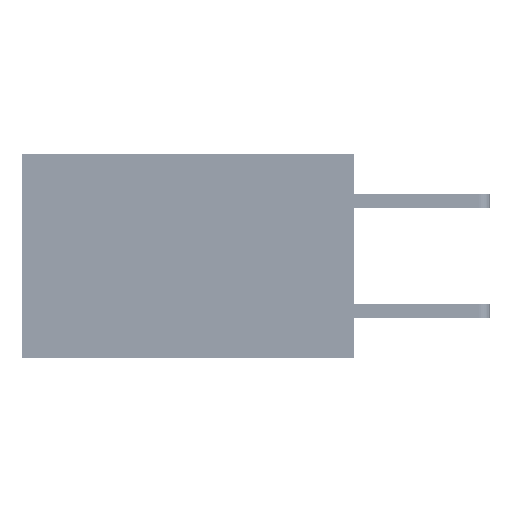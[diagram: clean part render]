
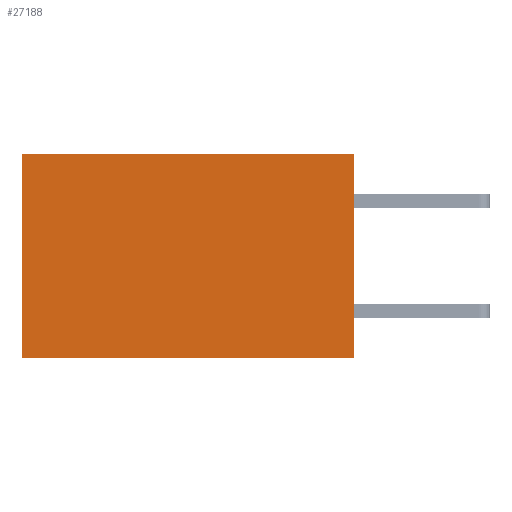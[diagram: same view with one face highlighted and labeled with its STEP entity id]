
A CAD part, left-side view. The second image highlights one B-rep face of the part: STEP entity #27188.
In plain terms, the highlighted planar face has unit normal (-1, 0, 0).
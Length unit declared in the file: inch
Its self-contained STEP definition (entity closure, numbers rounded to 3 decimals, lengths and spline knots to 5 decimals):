
#1308 = VERTEX_POINT ( 'NONE', #6621 ) ;
#3242 = DIRECTION ( 'NONE',  ( 0., 1., 0. ) ) ;
#3298 = VECTOR ( 'NONE', #3719, 39.37008 ) ;
#3719 = DIRECTION ( 'NONE',  ( 0., 1., 0. ) ) ;
#4143 = LINE ( 'NONE', #37745, #36942 ) ;
#4785 = VECTOR ( 'NONE', #3242, 39.37008 ) ;
#5758 = PLANE ( 'NONE',  #33249 ) ;
#6358 = LINE ( 'NONE', #19560, #4785 ) ;
#6621 = CARTESIAN_POINT ( 'NONE',  ( 0.2875, 0., 0. ) ) ;
#7656 = ORIENTED_EDGE ( 'NONE', *, *, #20569, .F. ) ;
#8825 = ORIENTED_EDGE ( 'NONE', *, *, #31269, .F. ) ;
#9727 = CARTESIAN_POINT ( 'NONE',  ( 0.2875, 0.6, -0.37 ) ) ;
#12631 = CARTESIAN_POINT ( 'NONE',  ( 0.2875, 0., 0. ) ) ;
#16343 = FACE_OUTER_BOUND ( 'NONE', #20433, .T. ) ;
#17646 = LINE ( 'NONE', #33254, #3298 ) ;
#17921 = EDGE_CURVE ( 'NONE', #32695, #18899, #24446, .T. ) ;
#18115 = DIRECTION ( 'NONE',  ( 0., 0., -1. ) ) ;
#18247 = VECTOR ( 'NONE', #21231, 39.37008 ) ;
#18899 = VERTEX_POINT ( 'NONE', #9727 ) ;
#19560 = CARTESIAN_POINT ( 'NONE',  ( 0.2875, 0., 0. ) ) ;
#20433 = EDGE_LOOP ( 'NONE', ( #25831, #8825, #7656, #35516 ) ) ;
#20569 = EDGE_CURVE ( 'NONE', #1308, #21246, #4143, .T. ) ;
#21231 = DIRECTION ( 'NONE',  ( 0., 0., -1. ) ) ;
#21246 = VERTEX_POINT ( 'NONE', #38425 ) ;
#22358 = DIRECTION ( 'NONE',  ( 1., 0., 0. ) ) ;
#24446 = LINE ( 'NONE', #40715, #18247 ) ;
#25831 = ORIENTED_EDGE ( 'NONE', *, *, #17921, .T. ) ;
#27188 = ADVANCED_FACE ( 'NONE', ( #16343 ), #5758, .F. ) ;
#31269 = EDGE_CURVE ( 'NONE', #21246, #18899, #17646, .T. ) ;
#31753 = EDGE_CURVE ( 'NONE', #1308, #32695, #6358, .T. ) ;
#32695 = VERTEX_POINT ( 'NONE', #33012 ) ;
#33012 = CARTESIAN_POINT ( 'NONE',  ( 0.2875, 0.6, 0. ) ) ;
#33249 = AXIS2_PLACEMENT_3D ( 'NONE', #12631, #22358, #41687 ) ;
#33254 = CARTESIAN_POINT ( 'NONE',  ( 0.2875, 0., -0.37 ) ) ;
#35516 = ORIENTED_EDGE ( 'NONE', *, *, #31753, .T. ) ;
#36942 = VECTOR ( 'NONE', #18115, 39.37008 ) ;
#37745 = CARTESIAN_POINT ( 'NONE',  ( 0.2875, 0., 0. ) ) ;
#38425 = CARTESIAN_POINT ( 'NONE',  ( 0.2875, 0., -0.37 ) ) ;
#40715 = CARTESIAN_POINT ( 'NONE',  ( 0.2875, 0.6, 0. ) ) ;
#41687 = DIRECTION ( 'NONE',  ( 0., 0., -1. ) ) ;
